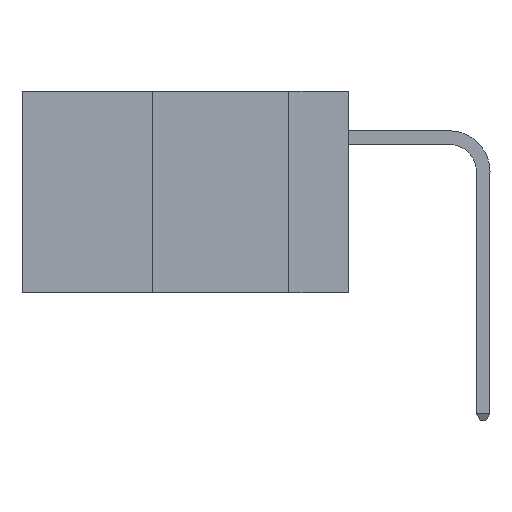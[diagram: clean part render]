
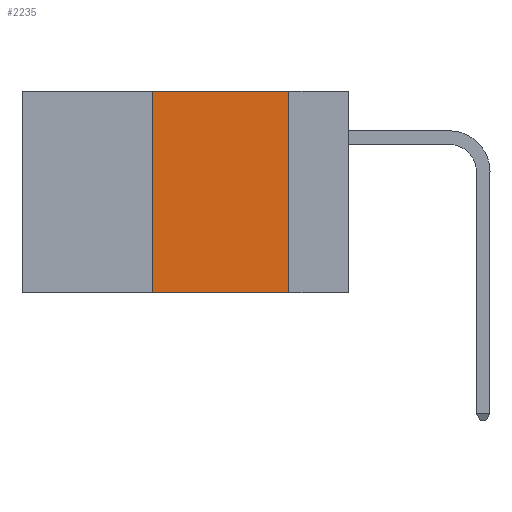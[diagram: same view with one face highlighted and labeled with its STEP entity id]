
A CAD part, left-side view. The second image highlights one B-rep face of the part: STEP entity #2235.
In plain terms, the highlighted planar face has unit normal (-1, 0, 0).
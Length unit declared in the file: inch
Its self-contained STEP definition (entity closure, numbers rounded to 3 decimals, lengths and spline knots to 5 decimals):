
#184 = LINE ( 'NONE', #10355, #6906 ) ;
#322 = CARTESIAN_POINT ( 'NONE',  ( 0., 0.11, -0.37 ) ) ;
#331 = CARTESIAN_POINT ( 'NONE',  ( 0., 0.11, 0. ) ) ;
#1209 = DIRECTION ( 'NONE',  ( 0., 0., 1. ) ) ;
#1320 = EDGE_CURVE ( 'NONE', #4863, #9497, #184, .T. ) ;
#1816 = CARTESIAN_POINT ( 'NONE',  ( 0., 0.11, 0. ) ) ;
#1896 = ORIENTED_EDGE ( 'NONE', *, *, #7542, .T. ) ;
#2002 = VERTEX_POINT ( 'NONE', #322 ) ;
#2235 = ADVANCED_FACE ( 'NONE', ( #5261 ), #8236, .F. ) ;
#2350 = LINE ( 'NONE', #4400, #9808 ) ;
#2571 = CARTESIAN_POINT ( 'NONE',  ( 0., 0.6, 0. ) ) ;
#3073 = VECTOR ( 'NONE', #8467, 39.37008 ) ;
#3500 = VECTOR ( 'NONE', #1209, 39.37008 ) ;
#3532 = DIRECTION ( 'NONE',  ( 0., 0., -1. ) ) ;
#4066 = CARTESIAN_POINT ( 'NONE',  ( 0., 0.36, -0.37 ) ) ;
#4400 = CARTESIAN_POINT ( 'NONE',  ( 0., 0.6, -0.37 ) ) ;
#4844 = DIRECTION ( 'NONE',  ( 0., -1., 0. ) ) ;
#4863 = VERTEX_POINT ( 'NONE', #9493 ) ;
#5054 = EDGE_LOOP ( 'NONE', ( #9093, #5486, #5781, #1896 ) ) ;
#5261 = FACE_OUTER_BOUND ( 'NONE', #5054, .T. ) ;
#5398 = EDGE_CURVE ( 'NONE', #9497, #2002, #5609, .T. ) ;
#5486 = ORIENTED_EDGE ( 'NONE', *, *, #1320, .F. ) ;
#5609 = LINE ( 'NONE', #1816, #3073 ) ;
#5781 = ORIENTED_EDGE ( 'NONE', *, *, #6736, .F. ) ;
#6046 = LINE ( 'NONE', #8580, #3500 ) ;
#6736 = EDGE_CURVE ( 'NONE', #10068, #4863, #6046, .T. ) ;
#6906 = VECTOR ( 'NONE', #4844, 39.37008 ) ;
#7542 = EDGE_CURVE ( 'NONE', #10068, #2002, #2350, .T. ) ;
#8236 = PLANE ( 'NONE',  #10301 ) ;
#8467 = DIRECTION ( 'NONE',  ( 0., 0., -1. ) ) ;
#8580 = CARTESIAN_POINT ( 'NONE',  ( 0., 0.36, 0. ) ) ;
#9093 = ORIENTED_EDGE ( 'NONE', *, *, #5398, .F. ) ;
#9137 = DIRECTION ( 'NONE',  ( 1., 0., 0. ) ) ;
#9493 = CARTESIAN_POINT ( 'NONE',  ( 0., 0.36, 0. ) ) ;
#9497 = VERTEX_POINT ( 'NONE', #331 ) ;
#9808 = VECTOR ( 'NONE', #10837, 39.37008 ) ;
#10068 = VERTEX_POINT ( 'NONE', #4066 ) ;
#10301 = AXIS2_PLACEMENT_3D ( 'NONE', #2571, #9137, #3532 ) ;
#10355 = CARTESIAN_POINT ( 'NONE',  ( 0., 0.6, 0. ) ) ;
#10837 = DIRECTION ( 'NONE',  ( 0., -1., 0. ) ) ;
